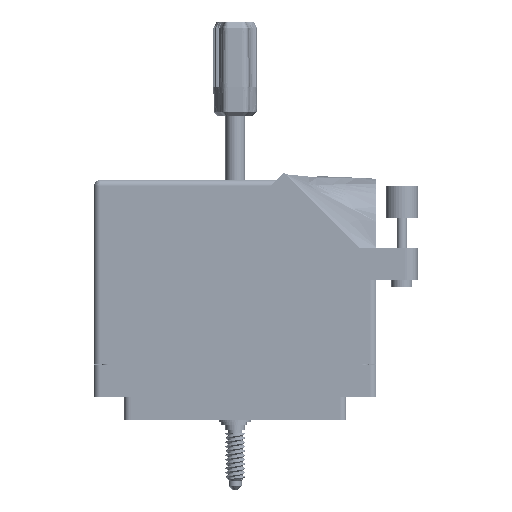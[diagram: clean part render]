
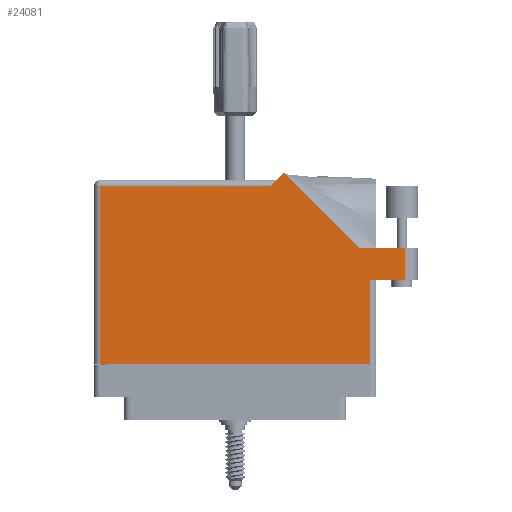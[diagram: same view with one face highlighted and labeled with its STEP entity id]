
A CAD part, front view. The second image highlights one B-rep face of the part: STEP entity #24081.
In plain terms, the highlighted face is planar.
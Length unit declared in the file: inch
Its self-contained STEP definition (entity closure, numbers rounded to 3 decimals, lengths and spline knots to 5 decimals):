
#1258 = VERTEX_POINT ( 'NONE', #22254 ) ;
#1912 = CARTESIAN_POINT ( 'NONE',  ( 1.19342, 1.022, 0.617 ) ) ;
#3787 = CARTESIAN_POINT ( 'NONE',  ( 1.634, 1.022, 0.617 ) ) ;
#4806 = CARTESIAN_POINT ( 'NONE',  ( 1.634, 1.022, 0.617 ) ) ;
#5140 = VECTOR ( 'NONE', #69036, 39.37008 ) ;
#5468 = CARTESIAN_POINT ( 'NONE',  ( -1.297, 1.613, 0.617 ) ) ;
#6998 = LINE ( 'NONE', #72492, #45871 ) ;
#9803 = VERTEX_POINT ( 'NONE', #75712 ) ;
#9878 = LINE ( 'NONE', #13009, #61211 ) ;
#12118 = DIRECTION ( 'NONE',  ( 1., 0., 0. ) ) ;
#12373 = VERTEX_POINT ( 'NONE', #5468 ) ;
#13009 = CARTESIAN_POINT ( 'NONE',  ( 1.359, 0.715, 0.617 ) ) ;
#14534 = DIRECTION ( 'NONE',  ( -0.707, -0.707, 0. ) ) ;
#16124 = FACE_OUTER_BOUND ( 'NONE', #57237, .T. ) ;
#16419 = VECTOR ( 'NONE', #19446, 39.37008 ) ;
#17120 = ORIENTED_EDGE ( 'NONE', *, *, #55579, .T. ) ;
#17804 = ORIENTED_EDGE ( 'NONE', *, *, #46873, .T. ) ;
#19446 = DIRECTION ( 'NONE',  ( 0., 1., 0. ) ) ;
#21914 = EDGE_CURVE ( 'NONE', #12373, #62741, #6998, .T. ) ;
#22254 = CARTESIAN_POINT ( 'NONE',  ( 1.19342, 1.022, 0.617 ) ) ;
#23746 = EDGE_CURVE ( 'NONE', #28225, #47651, #9878, .T. ) ;
#24081 = ADVANCED_FACE ( 'NONE', ( #16124 ), #77179, .F. ) ;
#24685 = CARTESIAN_POINT ( 'NONE',  ( 1.297, 0.715, 0.617 ) ) ;
#25417 = VERTEX_POINT ( 'NONE', #41755 ) ;
#27080 = ORIENTED_EDGE ( 'NONE', *, *, #23746, .T. ) ;
#27501 = CARTESIAN_POINT ( 'NONE',  ( 0.399, 1.675, 0.617 ) ) ;
#28225 = VERTEX_POINT ( 'NONE', #58308 ) ;
#30521 = DIRECTION ( 'NONE',  ( 0., 0., -1. ) ) ;
#31709 = ORIENTED_EDGE ( 'NONE', *, *, #61969, .T. ) ;
#31769 = VECTOR ( 'NONE', #14534, 39.37008 ) ;
#31895 = VECTOR ( 'NONE', #39053, 39.37008 ) ;
#33151 = CARTESIAN_POINT ( 'NONE',  ( 1.297, -0.1, 0.617 ) ) ;
#37886 = AXIS2_PLACEMENT_3D ( 'NONE', #70713, #30521, #77468 ) ;
#39052 = DIRECTION ( 'NONE',  ( 0., -1., 0. ) ) ;
#39053 = DIRECTION ( 'NONE',  ( 1., 0., 0. ) ) ;
#39096 = VECTOR ( 'NONE', #45765, 39.37008 ) ;
#41755 = CARTESIAN_POINT ( 'NONE',  ( 0.337, 1.613, 0.617 ) ) ;
#45765 = DIRECTION ( 'NONE',  ( 0., 1., 0. ) ) ;
#45871 = VECTOR ( 'NONE', #39052, 39.37008 ) ;
#45950 = EDGE_CURVE ( 'NONE', #58929, #1258, #86657, .T. ) ;
#46491 = DIRECTION ( 'NONE',  ( -1., 0., 0. ) ) ;
#46873 = EDGE_CURVE ( 'NONE', #62741, #70073, #51794, .T. ) ;
#47651 = VERTEX_POINT ( 'NONE', #82483 ) ;
#48574 = LINE ( 'NONE', #27501, #31769 ) ;
#50015 = ORIENTED_EDGE ( 'NONE', *, *, #63532, .T. ) ;
#51039 = LINE ( 'NONE', #4806, #16419 ) ;
#51794 = LINE ( 'NONE', #65707, #31895 ) ;
#52311 = ORIENTED_EDGE ( 'NONE', *, *, #45950, .T. ) ;
#52567 = EDGE_CURVE ( 'NONE', #70073, #28225, #56857, .T. ) ;
#54948 = DIRECTION ( 'NONE',  ( -1., 0., 0. ) ) ;
#55579 = EDGE_CURVE ( 'NONE', #9803, #25417, #48574, .T. ) ;
#56857 = LINE ( 'NONE', #24685, #39096 ) ;
#57237 = EDGE_LOOP ( 'NONE', ( #27080, #50015, #52311, #31709, #17120, #75763, #81946, #17804, #66303 ) ) ;
#58308 = CARTESIAN_POINT ( 'NONE',  ( 1.297, 0.715, 0.617 ) ) ;
#58929 = VERTEX_POINT ( 'NONE', #3787 ) ;
#59703 = LINE ( 'NONE', #1912, #5140 ) ;
#61211 = VECTOR ( 'NONE', #12118, 39.37008 ) ;
#61969 = EDGE_CURVE ( 'NONE', #1258, #9803, #59703, .T. ) ;
#62564 = VECTOR ( 'NONE', #54948, 39.37008 ) ;
#62741 = VERTEX_POINT ( 'NONE', #68422 ) ;
#63301 = EDGE_CURVE ( 'NONE', #25417, #12373, #85662, .T. ) ;
#63532 = EDGE_CURVE ( 'NONE', #47651, #58929, #51039, .T. ) ;
#64633 = VECTOR ( 'NONE', #46491, 39.37008 ) ;
#65707 = CARTESIAN_POINT ( 'NONE',  ( -1.359, -0.1, 0.617 ) ) ;
#66144 = CARTESIAN_POINT ( 'NONE',  ( 1.759, 1.022, 0.617 ) ) ;
#66303 = ORIENTED_EDGE ( 'NONE', *, *, #52567, .T. ) ;
#68422 = CARTESIAN_POINT ( 'NONE',  ( -1.297, -0.1, 0.617 ) ) ;
#69036 = DIRECTION ( 'NONE',  ( -0.707, 0.707, 0. ) ) ;
#70073 = VERTEX_POINT ( 'NONE', #33151 ) ;
#70713 = CARTESIAN_POINT ( 'NONE',  ( -1.359, 1.675, 0.617 ) ) ;
#72492 = CARTESIAN_POINT ( 'NONE',  ( -1.297, -0.1, 0.617 ) ) ;
#72959 = CARTESIAN_POINT ( 'NONE',  ( -1.359, 1.613, 0.617 ) ) ;
#75712 = CARTESIAN_POINT ( 'NONE',  ( 0.46971, 1.74571, 0.617 ) ) ;
#75763 = ORIENTED_EDGE ( 'NONE', *, *, #63301, .T. ) ;
#77179 = PLANE ( 'NONE',  #37886 ) ;
#77468 = DIRECTION ( 'NONE',  ( -1., 0., 0. ) ) ;
#81946 = ORIENTED_EDGE ( 'NONE', *, *, #21914, .T. ) ;
#82483 = CARTESIAN_POINT ( 'NONE',  ( 1.634, 0.715, 0.617 ) ) ;
#85662 = LINE ( 'NONE', #72959, #62564 ) ;
#86657 = LINE ( 'NONE', #66144, #64633 ) ;
